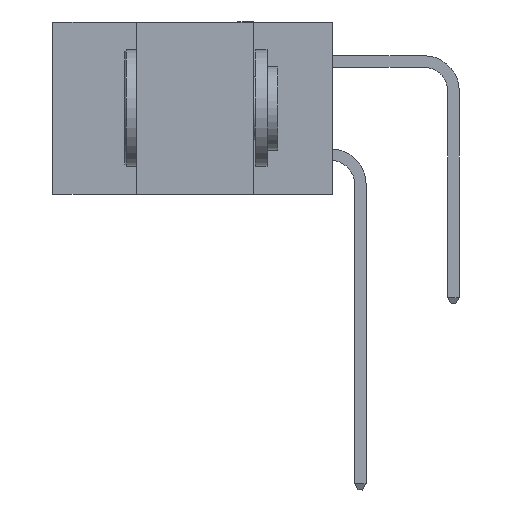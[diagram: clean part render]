
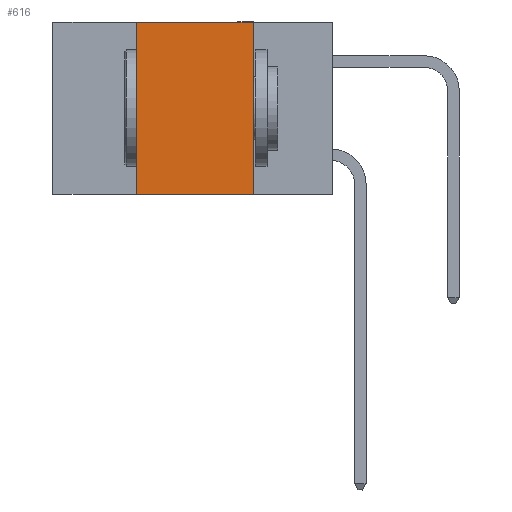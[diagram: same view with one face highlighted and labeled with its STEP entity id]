
A CAD part, left-side view. The second image highlights one B-rep face of the part: STEP entity #616.
In plain terms, the highlighted planar face has unit normal (-1, 0, 0).
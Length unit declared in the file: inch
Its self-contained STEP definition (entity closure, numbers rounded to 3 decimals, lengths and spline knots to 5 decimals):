
#215 = LINE ( 'NONE', #7712, #11497 ) ;
#616 = ADVANCED_FACE ( 'NONE', ( #6278 ), #11743, .F. ) ;
#888 = CARTESIAN_POINT ( 'NONE',  ( 0., 0.42, 0. ) ) ;
#3057 = DIRECTION ( 'NONE',  ( 1., 0., 0. ) ) ;
#3389 = EDGE_CURVE ( 'NONE', #5440, #13023, #215, .T. ) ;
#3419 = EDGE_CURVE ( 'NONE', #13023, #10499, #7111, .T. ) ;
#3678 = VECTOR ( 'NONE', #14238, 39.37008 ) ;
#4572 = CARTESIAN_POINT ( 'NONE',  ( 0., 0.17, 0. ) ) ;
#5120 = EDGE_CURVE ( 'NONE', #10098, #5440, #16246, .T. ) ;
#5440 = VERTEX_POINT ( 'NONE', #5595 ) ;
#5595 = CARTESIAN_POINT ( 'NONE',  ( 0., 0.42, 0. ) ) ;
#6278 = FACE_OUTER_BOUND ( 'NONE', #6980, .T. ) ;
#6980 = EDGE_LOOP ( 'NONE', ( #18986, #9196, #16097, #10618 ) ) ;
#7111 = LINE ( 'NONE', #4572, #3678 ) ;
#7168 = DIRECTION ( 'NONE',  ( 0., 0., 1. ) ) ;
#7517 = LINE ( 'NONE', #12026, #18300 ) ;
#7712 = CARTESIAN_POINT ( 'NONE',  ( 0., 0.6, 0. ) ) ;
#8504 = DIRECTION ( 'NONE',  ( 0., -1., 0. ) ) ;
#9196 = ORIENTED_EDGE ( 'NONE', *, *, #3389, .F. ) ;
#10098 = VERTEX_POINT ( 'NONE', #12993 ) ;
#10499 = VERTEX_POINT ( 'NONE', #10946 ) ;
#10618 = ORIENTED_EDGE ( 'NONE', *, *, #18270, .T. ) ;
#10946 = CARTESIAN_POINT ( 'NONE',  ( 0., 0.17, -0.37 ) ) ;
#11408 = CARTESIAN_POINT ( 'NONE',  ( 0., 0.6, 0. ) ) ;
#11497 = VECTOR ( 'NONE', #8504, 39.37008 ) ;
#11565 = DIRECTION ( 'NONE',  ( 0., 0., -1. ) ) ;
#11743 = PLANE ( 'NONE',  #16605 ) ;
#12026 = CARTESIAN_POINT ( 'NONE',  ( 0., 0.6, -0.37 ) ) ;
#12993 = CARTESIAN_POINT ( 'NONE',  ( 0., 0.42, -0.37 ) ) ;
#13023 = VERTEX_POINT ( 'NONE', #16213 ) ;
#13519 = DIRECTION ( 'NONE',  ( 0., -1., 0. ) ) ;
#14238 = DIRECTION ( 'NONE',  ( 0., 0., -1. ) ) ;
#15798 = VECTOR ( 'NONE', #7168, 39.37008 ) ;
#16097 = ORIENTED_EDGE ( 'NONE', *, *, #5120, .F. ) ;
#16213 = CARTESIAN_POINT ( 'NONE',  ( 0., 0.17, 0. ) ) ;
#16246 = LINE ( 'NONE', #888, #15798 ) ;
#16605 = AXIS2_PLACEMENT_3D ( 'NONE', #11408, #3057, #11565 ) ;
#18270 = EDGE_CURVE ( 'NONE', #10098, #10499, #7517, .T. ) ;
#18300 = VECTOR ( 'NONE', #13519, 39.37008 ) ;
#18986 = ORIENTED_EDGE ( 'NONE', *, *, #3419, .F. ) ;
